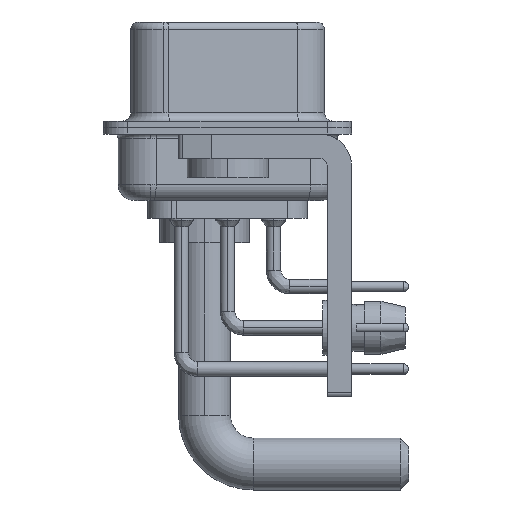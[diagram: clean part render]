
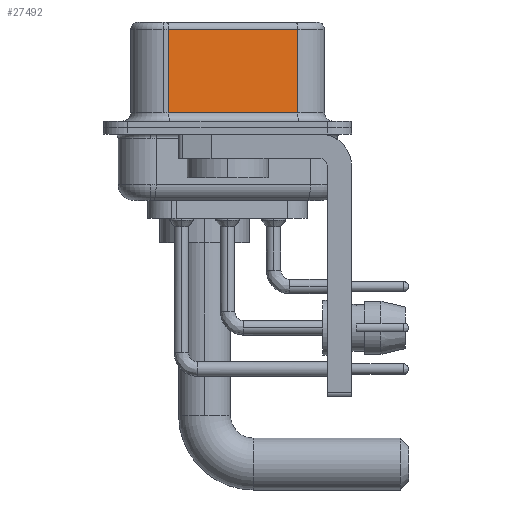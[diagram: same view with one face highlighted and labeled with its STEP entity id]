
A CAD part, left-side view. The second image highlights one B-rep face of the part: STEP entity #27492.
In plain terms, the highlighted planar face has unit normal (-0.985, -0.174, 0).
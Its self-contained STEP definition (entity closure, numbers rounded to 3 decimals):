
#37 = PLANE ( 'NONE',  #38335 ) ;
#1341 = CARTESIAN_POINT ( 'NONE',  ( 5.132, -4.322, 6.02 ) ) ;
#2112 = EDGE_CURVE ( 'NONE', #2171, #11953, #36532, .T. ) ;
#2171 = VERTEX_POINT ( 'NONE', #2477 ) ;
#2477 = CARTESIAN_POINT ( 'NONE',  ( 3.73, 3.628, 0.9 ) ) ;
#4315 = CARTESIAN_POINT ( 'NONE',  ( 3.73, 3.628, 6.02 ) ) ;
#6937 = CARTESIAN_POINT ( 'NONE',  ( 5.132, -4.322, 6.52 ) ) ;
#6943 = DIRECTION ( 'NONE',  ( -0.174, 0.985, 0. ) ) ;
#7195 = CARTESIAN_POINT ( 'NONE',  ( 3.73, 3.628, 6.52 ) ) ;
#8345 = DIRECTION ( 'NONE',  ( 0.174, -0.985, 0. ) ) ;
#8950 = ORIENTED_EDGE ( 'NONE', *, *, #33336, .F. ) ;
#9818 = CARTESIAN_POINT ( 'NONE',  ( 5.132, -4.322, 6.52 ) ) ;
#10051 = EDGE_CURVE ( 'NONE', #18819, #17000, #12418, .T. ) ;
#11001 = VECTOR ( 'NONE', #8345, 1000. ) ;
#11146 = VECTOR ( 'NONE', #34469, 1000. ) ;
#11953 = VERTEX_POINT ( 'NONE', #28691 ) ;
#12055 = ORIENTED_EDGE ( 'NONE', *, *, #10051, .T. ) ;
#12098 = EDGE_LOOP ( 'NONE', ( #8950, #12055, #25258, #12276 ) ) ;
#12220 = CARTESIAN_POINT ( 'NONE',  ( 5.132, -4.322, 6.02 ) ) ;
#12276 = ORIENTED_EDGE ( 'NONE', *, *, #2112, .T. ) ;
#12418 = LINE ( 'NONE', #12220, #29391 ) ;
#15324 = DIRECTION ( 'NONE',  ( 0.985, 0.174, 0. ) ) ;
#17000 = VERTEX_POINT ( 'NONE', #4315 ) ;
#18819 = VERTEX_POINT ( 'NONE', #1341 ) ;
#21020 = FACE_OUTER_BOUND ( 'NONE', #12098, .T. ) ;
#24481 = VECTOR ( 'NONE', #33444, 1000. ) ;
#24985 = LINE ( 'NONE', #6937, #24481 ) ;
#25258 = ORIENTED_EDGE ( 'NONE', *, *, #29483, .T. ) ;
#27492 = ADVANCED_FACE ( 'NONE', ( #21020 ), #37, .F. ) ;
#28691 = CARTESIAN_POINT ( 'NONE',  ( 5.132, -4.322, 0.9 ) ) ;
#29391 = VECTOR ( 'NONE', #6943, 1000. ) ;
#29483 = EDGE_CURVE ( 'NONE', #17000, #2171, #37231, .T. ) ;
#32693 = CARTESIAN_POINT ( 'NONE',  ( 5.132, -4.322, 0.9 ) ) ;
#33015 = DIRECTION ( 'NONE',  ( -0.174, 0.985, 0. ) ) ;
#33336 = EDGE_CURVE ( 'NONE', #18819, #11953, #24985, .T. ) ;
#33444 = DIRECTION ( 'NONE',  ( 0., 0., -1. ) ) ;
#34469 = DIRECTION ( 'NONE',  ( 0., 0., -1. ) ) ;
#36532 = LINE ( 'NONE', #32693, #11001 ) ;
#37231 = LINE ( 'NONE', #7195, #11146 ) ;
#38335 = AXIS2_PLACEMENT_3D ( 'NONE', #9818, #15324, #33015 ) ;
